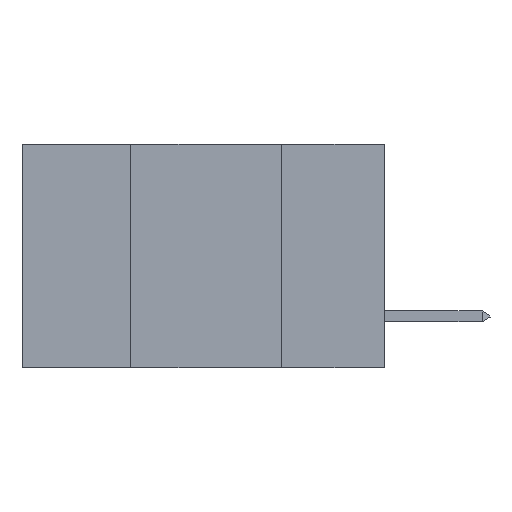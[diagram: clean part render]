
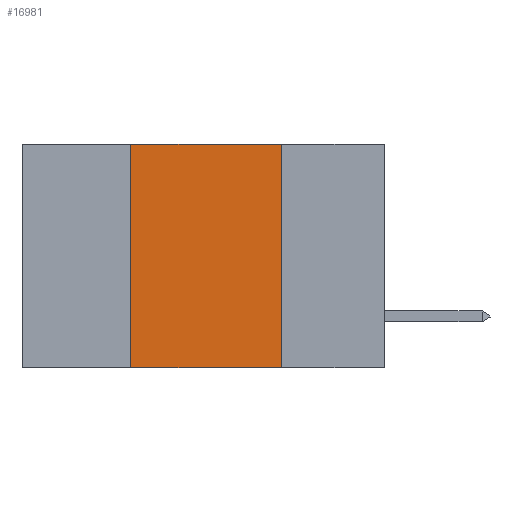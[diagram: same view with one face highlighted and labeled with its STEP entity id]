
A CAD part, left-side view. The second image highlights one B-rep face of the part: STEP entity #16981.
In plain terms, the highlighted planar face has unit normal (-1, 0, 0).
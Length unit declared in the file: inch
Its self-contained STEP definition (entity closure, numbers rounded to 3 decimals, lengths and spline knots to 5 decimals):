
#1869 = ORIENTED_EDGE ( 'NONE', *, *, #30280, .F. ) ;
#3095 = FACE_OUTER_BOUND ( 'NONE', #8553, .T. ) ;
#4182 = DIRECTION ( 'NONE',  ( 0., -1., 0. ) ) ;
#5468 = DIRECTION ( 'NONE',  ( 1., 0., 0. ) ) ;
#5804 = CARTESIAN_POINT ( 'NONE',  ( 0., 0.42, 0. ) ) ;
#5960 = DIRECTION ( 'NONE',  ( 0., 0., -1. ) ) ;
#7795 = VERTEX_POINT ( 'NONE', #39198 ) ;
#8553 = EDGE_LOOP ( 'NONE', ( #21295, #29119, #1869, #15719 ) ) ;
#11061 = DIRECTION ( 'NONE',  ( 0., -1., 0. ) ) ;
#12183 = DIRECTION ( 'NONE',  ( 0., 0., -1. ) ) ;
#12814 = CARTESIAN_POINT ( 'NONE',  ( 0., 0.17, 0. ) ) ;
#13745 = VECTOR ( 'NONE', #4182, 39.37008 ) ;
#15719 = ORIENTED_EDGE ( 'NONE', *, *, #41333, .T. ) ;
#15909 = VECTOR ( 'NONE', #11061, 39.37008 ) ;
#16383 = DIRECTION ( 'NONE',  ( 0., 0., 1. ) ) ;
#16981 = ADVANCED_FACE ( 'NONE', ( #3095 ), #42792, .F. ) ;
#17947 = LINE ( 'NONE', #34794, #13745 ) ;
#18039 = CARTESIAN_POINT ( 'NONE',  ( 0., 0.6, -0.37 ) ) ;
#21272 = VECTOR ( 'NONE', #5960, 39.37008 ) ;
#21295 = ORIENTED_EDGE ( 'NONE', *, *, #40446, .F. ) ;
#26114 = VERTEX_POINT ( 'NONE', #28360 ) ;
#27207 = LINE ( 'NONE', #12814, #21272 ) ;
#28360 = CARTESIAN_POINT ( 'NONE',  ( 0., 0.17, -0.37 ) ) ;
#29117 = CARTESIAN_POINT ( 'NONE',  ( 0., 0.42, -0.37 ) ) ;
#29119 = ORIENTED_EDGE ( 'NONE', *, *, #31153, .F. ) ;
#30280 = EDGE_CURVE ( 'NONE', #43943, #7795, #38389, .T. ) ;
#31153 = EDGE_CURVE ( 'NONE', #7795, #43326, #17947, .T. ) ;
#32627 = CARTESIAN_POINT ( 'NONE',  ( 0., 0.6, 0. ) ) ;
#34113 = LINE ( 'NONE', #18039, #15909 ) ;
#34275 = AXIS2_PLACEMENT_3D ( 'NONE', #32627, #5468, #12183 ) ;
#34794 = CARTESIAN_POINT ( 'NONE',  ( 0., 0.6, 0. ) ) ;
#38389 = LINE ( 'NONE', #5804, #39461 ) ;
#39198 = CARTESIAN_POINT ( 'NONE',  ( 0., 0.42, 0. ) ) ;
#39461 = VECTOR ( 'NONE', #16383, 39.37008 ) ;
#40446 = EDGE_CURVE ( 'NONE', #43326, #26114, #27207, .T. ) ;
#41333 = EDGE_CURVE ( 'NONE', #43943, #26114, #34113, .T. ) ;
#42630 = CARTESIAN_POINT ( 'NONE',  ( 0., 0.17, 0. ) ) ;
#42792 = PLANE ( 'NONE',  #34275 ) ;
#43326 = VERTEX_POINT ( 'NONE', #42630 ) ;
#43943 = VERTEX_POINT ( 'NONE', #29117 ) ;
